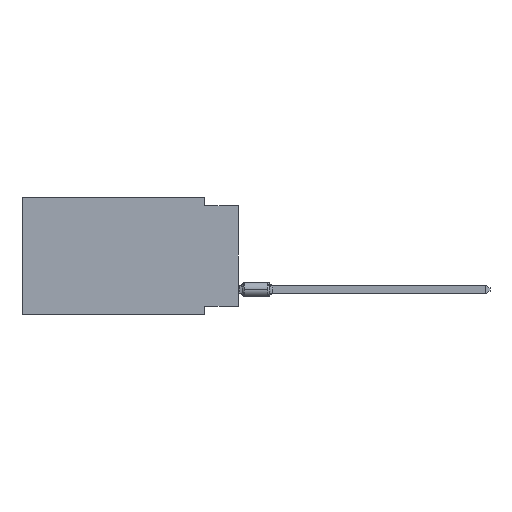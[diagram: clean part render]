
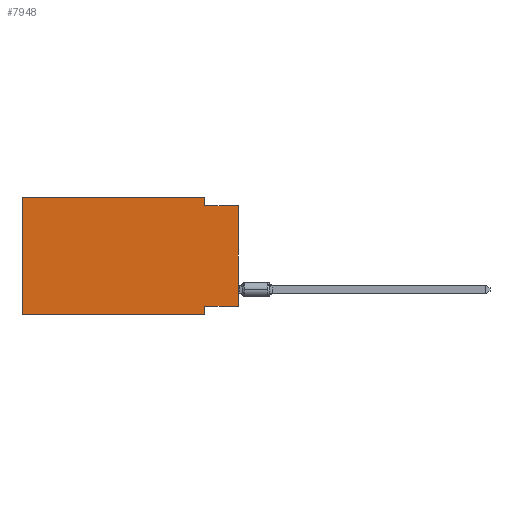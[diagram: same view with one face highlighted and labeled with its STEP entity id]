
A CAD part, left-side view. The second image highlights one B-rep face of the part: STEP entity #7948.
In plain terms, the highlighted planar face has unit normal (-1, 0, 0).
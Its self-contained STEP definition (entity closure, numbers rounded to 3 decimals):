
#309 = VERTEX_POINT ( 'NONE', #18200 ) ;
#382 = DIRECTION ( 'NONE',  ( 0., 0., -1. ) ) ;
#448 = CARTESIAN_POINT ( 'NONE',  ( 0., 2.54, -8.89 ) ) ;
#701 = DIRECTION ( 'NONE',  ( 0., 1., 0. ) ) ;
#976 = VECTOR ( 'NONE', #382, 1000. ) ;
#1192 = VERTEX_POINT ( 'NONE', #6358 ) ;
#1925 = EDGE_CURVE ( 'NONE', #1192, #5563, #6514, .T. ) ;
#2528 = CARTESIAN_POINT ( 'NONE',  ( 0., 16.383, 0. ) ) ;
#2569 = CARTESIAN_POINT ( 'NONE',  ( 0., 2.54, -8.89 ) ) ;
#4163 = ORIENTED_EDGE ( 'NONE', *, *, #10209, .F. ) ;
#4348 = VERTEX_POINT ( 'NONE', #20547 ) ;
#5533 = VECTOR ( 'NONE', #22352, 1000. ) ;
#5563 = VERTEX_POINT ( 'NONE', #448 ) ;
#5837 = EDGE_CURVE ( 'NONE', #10465, #309, #24951, .T. ) ;
#6358 = CARTESIAN_POINT ( 'NONE',  ( 0., 2.54, -8.255 ) ) ;
#6362 = ORIENTED_EDGE ( 'NONE', *, *, #9950, .T. ) ;
#6391 = CARTESIAN_POINT ( 'NONE',  ( 0., 0., 0. ) ) ;
#6433 = AXIS2_PLACEMENT_3D ( 'NONE', #8770, #10686, #23494 ) ;
#6514 = LINE ( 'NONE', #2569, #976 ) ;
#7564 = VECTOR ( 'NONE', #8162, 1000. ) ;
#7686 = ORIENTED_EDGE ( 'NONE', *, *, #9915, .F. ) ;
#7948 = ADVANCED_FACE ( 'NONE', ( #15180 ), #21046, .F. ) ;
#8162 = DIRECTION ( 'NONE',  ( 0., -1., 0. ) ) ;
#8174 = DIRECTION ( 'NONE',  ( 0., 0., -1. ) ) ;
#8563 = LINE ( 'NONE', #6391, #15836 ) ;
#8770 = CARTESIAN_POINT ( 'NONE',  ( 0., 16.383, 0. ) ) ;
#9208 = EDGE_CURVE ( 'NONE', #22547, #1192, #23460, .T. ) ;
#9320 = CARTESIAN_POINT ( 'NONE',  ( 0., 2.54, 0. ) ) ;
#9330 = VECTOR ( 'NONE', #16737, 1000. ) ;
#9652 = DIRECTION ( 'NONE',  ( 0., 0., 1. ) ) ;
#9915 = EDGE_CURVE ( 'NONE', #21691, #10465, #25070, .T. ) ;
#9950 = EDGE_CURVE ( 'NONE', #22547, #18324, #8563, .T. ) ;
#10209 = EDGE_CURVE ( 'NONE', #4348, #21691, #26153, .T. ) ;
#10465 = VERTEX_POINT ( 'NONE', #9320 ) ;
#10686 = DIRECTION ( 'NONE',  ( 1., 0., 0. ) ) ;
#12899 = LINE ( 'NONE', #21224, #9330 ) ;
#13100 = CARTESIAN_POINT ( 'NONE',  ( 0., 0., -8.255 ) ) ;
#14179 = CARTESIAN_POINT ( 'NONE',  ( 0., 2.54, 0. ) ) ;
#14303 = DIRECTION ( 'NONE',  ( 0., 0., 1. ) ) ;
#14775 = CARTESIAN_POINT ( 'NONE',  ( 0., 0., -0.635 ) ) ;
#15180 = FACE_OUTER_BOUND ( 'NONE', #20272, .T. ) ;
#15836 = VECTOR ( 'NONE', #14303, 1000. ) ;
#16737 = DIRECTION ( 'NONE',  ( 0., -1., 0. ) ) ;
#17230 = EDGE_CURVE ( 'NONE', #4348, #5563, #26698, .T. ) ;
#17356 = ORIENTED_EDGE ( 'NONE', *, *, #17230, .T. ) ;
#18104 = CARTESIAN_POINT ( 'NONE',  ( 0., 16.383, 0. ) ) ;
#18200 = CARTESIAN_POINT ( 'NONE',  ( 0., 2.54, -0.635 ) ) ;
#18324 = VERTEX_POINT ( 'NONE', #14775 ) ;
#20272 = EDGE_LOOP ( 'NONE', ( #6362, #20940, #21640, #7686, #4163, #17356, #24812, #22265 ) ) ;
#20547 = CARTESIAN_POINT ( 'NONE',  ( 0., 16.383, -8.89 ) ) ;
#20579 = CARTESIAN_POINT ( 'NONE',  ( 0., 16.383, 0. ) ) ;
#20677 = VECTOR ( 'NONE', #701, 1000. ) ;
#20940 = ORIENTED_EDGE ( 'NONE', *, *, #24884, .F. ) ;
#21046 = PLANE ( 'NONE',  #6433 ) ;
#21224 = CARTESIAN_POINT ( 'NONE',  ( 0., 0., -0.635 ) ) ;
#21640 = ORIENTED_EDGE ( 'NONE', *, *, #5837, .F. ) ;
#21691 = VERTEX_POINT ( 'NONE', #2528 ) ;
#22265 = ORIENTED_EDGE ( 'NONE', *, *, #9208, .F. ) ;
#22352 = DIRECTION ( 'NONE',  ( 0., -1., 0. ) ) ;
#22547 = VERTEX_POINT ( 'NONE', #25770 ) ;
#22777 = VECTOR ( 'NONE', #9652, 1000. ) ;
#23460 = LINE ( 'NONE', #13100, #20677 ) ;
#23494 = DIRECTION ( 'NONE',  ( 0., 0., -1. ) ) ;
#24251 = CARTESIAN_POINT ( 'NONE',  ( 0., 16.383, -8.89 ) ) ;
#24643 = VECTOR ( 'NONE', #8174, 1000. ) ;
#24812 = ORIENTED_EDGE ( 'NONE', *, *, #1925, .F. ) ;
#24884 = EDGE_CURVE ( 'NONE', #309, #18324, #12899, .T. ) ;
#24951 = LINE ( 'NONE', #14179, #24643 ) ;
#25070 = LINE ( 'NONE', #20579, #7564 ) ;
#25770 = CARTESIAN_POINT ( 'NONE',  ( 0., 0., -8.255 ) ) ;
#26153 = LINE ( 'NONE', #18104, #22777 ) ;
#26698 = LINE ( 'NONE', #24251, #5533 ) ;
